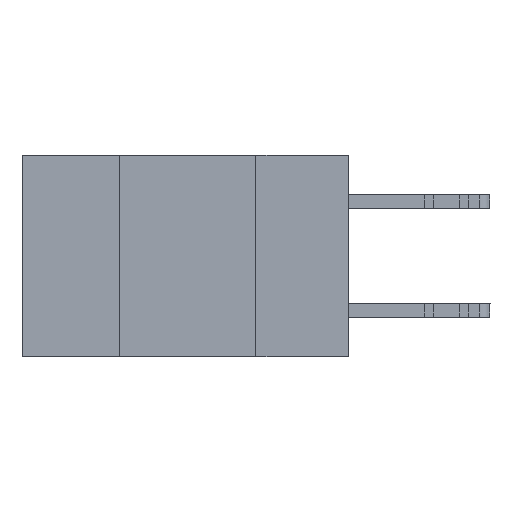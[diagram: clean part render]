
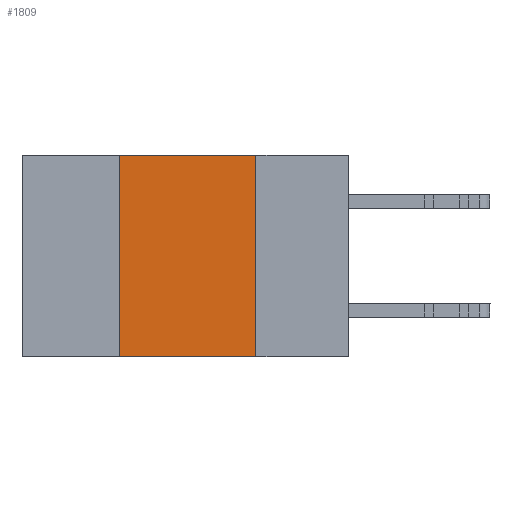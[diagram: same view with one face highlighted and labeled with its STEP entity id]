
A CAD part, left-side view. The second image highlights one B-rep face of the part: STEP entity #1809.
In plain terms, the highlighted planar face has unit normal (-1, 0, 0).
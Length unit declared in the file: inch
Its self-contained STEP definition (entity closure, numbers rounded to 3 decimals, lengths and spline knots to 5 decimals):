
#767 = CARTESIAN_POINT ( 'NONE',  ( 0., 0.42, -0.37 ) ) ;
#994 = AXIS2_PLACEMENT_3D ( 'NONE', #13671, #11056, #13641 ) ;
#1809 = ADVANCED_FACE ( 'NONE', ( #12196 ), #10897, .F. ) ;
#2302 = DIRECTION ( 'NONE',  ( 0., -1., 0. ) ) ;
#2418 = VECTOR ( 'NONE', #2302, 39.37008 ) ;
#3185 = CARTESIAN_POINT ( 'NONE',  ( 0., 0.42, 0. ) ) ;
#3569 = VERTEX_POINT ( 'NONE', #6237 ) ;
#4489 = CARTESIAN_POINT ( 'NONE',  ( 0., 0.42, -0.37 ) ) ;
#5743 = VERTEX_POINT ( 'NONE', #3185 ) ;
#5785 = VECTOR ( 'NONE', #6423, 39.37008 ) ;
#6093 = VECTOR ( 'NONE', #7944, 39.37008 ) ;
#6237 = CARTESIAN_POINT ( 'NONE',  ( 0., 0.17, 0. ) ) ;
#6299 = DIRECTION ( 'NONE',  ( 0., -1., 0. ) ) ;
#6423 = DIRECTION ( 'NONE',  ( 0., 0., 1. ) ) ;
#7415 = ORIENTED_EDGE ( 'NONE', *, *, #15693, .F. ) ;
#7944 = DIRECTION ( 'NONE',  ( 0., 0., -1. ) ) ;
#10897 = PLANE ( 'NONE',  #994 ) ;
#11056 = DIRECTION ( 'NONE',  ( 1., 0., 0. ) ) ;
#12109 = EDGE_LOOP ( 'NONE', ( #7415, #17649, #22402, #13982 ) ) ;
#12122 = LINE ( 'NONE', #15070, #2418 ) ;
#12196 = FACE_OUTER_BOUND ( 'NONE', #12109, .T. ) ;
#13641 = DIRECTION ( 'NONE',  ( 0., 0., -1. ) ) ;
#13671 = CARTESIAN_POINT ( 'NONE',  ( 0., 0.6, 0. ) ) ;
#13982 = ORIENTED_EDGE ( 'NONE', *, *, #19285, .T. ) ;
#14278 = LINE ( 'NONE', #22584, #14841 ) ;
#14841 = VECTOR ( 'NONE', #6299, 39.37008 ) ;
#15070 = CARTESIAN_POINT ( 'NONE',  ( 0., 0.6, 0. ) ) ;
#15693 = EDGE_CURVE ( 'NONE', #3569, #20985, #16349, .T. ) ;
#16349 = LINE ( 'NONE', #18813, #6093 ) ;
#16897 = EDGE_CURVE ( 'NONE', #5743, #3569, #12122, .T. ) ;
#17649 = ORIENTED_EDGE ( 'NONE', *, *, #16897, .F. ) ;
#18087 = EDGE_CURVE ( 'NONE', #21685, #5743, #20265, .T. ) ;
#18813 = CARTESIAN_POINT ( 'NONE',  ( 0., 0.17, -0.37 ) ) ;
#19061 = CARTESIAN_POINT ( 'NONE',  ( 0., 0.17, -0.37 ) ) ;
#19285 = EDGE_CURVE ( 'NONE', #21685, #20985, #14278, .T. ) ;
#20265 = LINE ( 'NONE', #767, #5785 ) ;
#20985 = VERTEX_POINT ( 'NONE', #19061 ) ;
#21685 = VERTEX_POINT ( 'NONE', #4489 ) ;
#22402 = ORIENTED_EDGE ( 'NONE', *, *, #18087, .F. ) ;
#22584 = CARTESIAN_POINT ( 'NONE',  ( 0., 0.6, -0.37 ) ) ;
